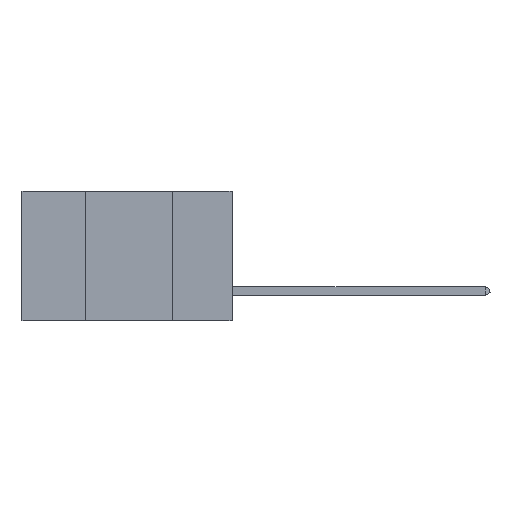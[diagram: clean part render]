
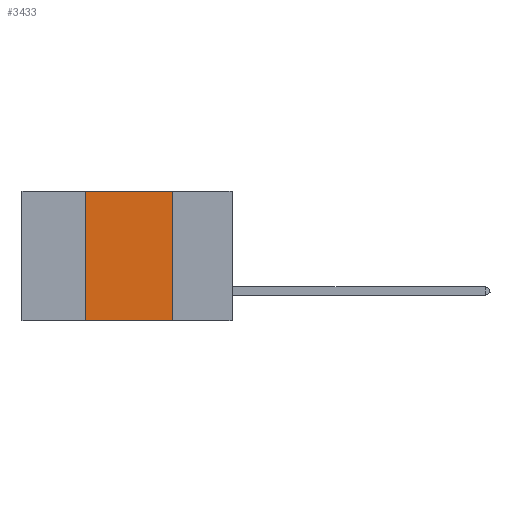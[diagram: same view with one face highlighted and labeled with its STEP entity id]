
A CAD part, left-side view. The second image highlights one B-rep face of the part: STEP entity #3433.
In plain terms, the highlighted planar face has unit normal (-1, 0, 0).
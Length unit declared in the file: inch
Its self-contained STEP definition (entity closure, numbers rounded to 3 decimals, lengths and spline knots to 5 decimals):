
#653 = CARTESIAN_POINT ( 'NONE',  ( 0., 0.6, 0. ) ) ;
#1220 = EDGE_CURVE ( 'NONE', #8107, #5105, #1917, .T. ) ;
#1450 = FACE_OUTER_BOUND ( 'NONE', #9660, .T. ) ;
#1591 = EDGE_CURVE ( 'NONE', #3812, #8107, #2342, .T. ) ;
#1629 = EDGE_CURVE ( 'NONE', #3812, #6533, #5517, .T. ) ;
#1671 = CARTESIAN_POINT ( 'NONE',  ( 0., 0.42, 0. ) ) ;
#1917 = LINE ( 'NONE', #6794, #5126 ) ;
#2342 = LINE ( 'NONE', #4908, #3270 ) ;
#3156 = DIRECTION ( 'NONE',  ( 0., 0., -1. ) ) ;
#3270 = VECTOR ( 'NONE', #6660, 39.37008 ) ;
#3370 = DIRECTION ( 'NONE',  ( 0., -1., 0. ) ) ;
#3433 = ADVANCED_FACE ( 'NONE', ( #1450 ), #4903, .F. ) ;
#3536 = VECTOR ( 'NONE', #5535, 39.37008 ) ;
#3812 = VERTEX_POINT ( 'NONE', #5273 ) ;
#4903 = PLANE ( 'NONE',  #6041 ) ;
#4908 = CARTESIAN_POINT ( 'NONE',  ( 0., 0.42, 0. ) ) ;
#5105 = VERTEX_POINT ( 'NONE', #5284 ) ;
#5126 = VECTOR ( 'NONE', #10250, 39.37008 ) ;
#5174 = CARTESIAN_POINT ( 'NONE',  ( 0., 0.6, -0.37 ) ) ;
#5273 = CARTESIAN_POINT ( 'NONE',  ( 0., 0.42, -0.37 ) ) ;
#5284 = CARTESIAN_POINT ( 'NONE',  ( 0., 0.17, 0. ) ) ;
#5517 = LINE ( 'NONE', #5174, #9843 ) ;
#5535 = DIRECTION ( 'NONE',  ( 0., 0., -1. ) ) ;
#5734 = CARTESIAN_POINT ( 'NONE',  ( 0., 0.17, -0.37 ) ) ;
#5942 = ORIENTED_EDGE ( 'NONE', *, *, #1591, .F. ) ;
#6041 = AXIS2_PLACEMENT_3D ( 'NONE', #653, #7484, #3156 ) ;
#6187 = LINE ( 'NONE', #9917, #3536 ) ;
#6533 = VERTEX_POINT ( 'NONE', #5734 ) ;
#6602 = ORIENTED_EDGE ( 'NONE', *, *, #7087, .F. ) ;
#6660 = DIRECTION ( 'NONE',  ( 0., 0., 1. ) ) ;
#6794 = CARTESIAN_POINT ( 'NONE',  ( 0., 0.6, 0. ) ) ;
#7087 = EDGE_CURVE ( 'NONE', #5105, #6533, #6187, .T. ) ;
#7484 = DIRECTION ( 'NONE',  ( 1., 0., 0. ) ) ;
#8041 = ORIENTED_EDGE ( 'NONE', *, *, #1220, .F. ) ;
#8107 = VERTEX_POINT ( 'NONE', #1671 ) ;
#8202 = ORIENTED_EDGE ( 'NONE', *, *, #1629, .T. ) ;
#9660 = EDGE_LOOP ( 'NONE', ( #6602, #8041, #5942, #8202 ) ) ;
#9843 = VECTOR ( 'NONE', #3370, 39.37008 ) ;
#9917 = CARTESIAN_POINT ( 'NONE',  ( 0., 0.17, 0. ) ) ;
#10250 = DIRECTION ( 'NONE',  ( 0., -1., 0. ) ) ;
